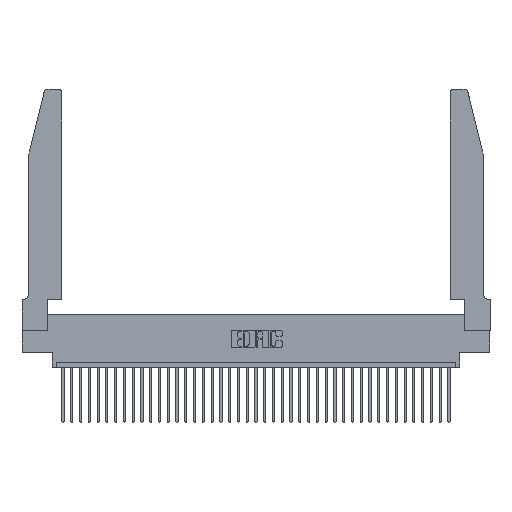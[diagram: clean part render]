
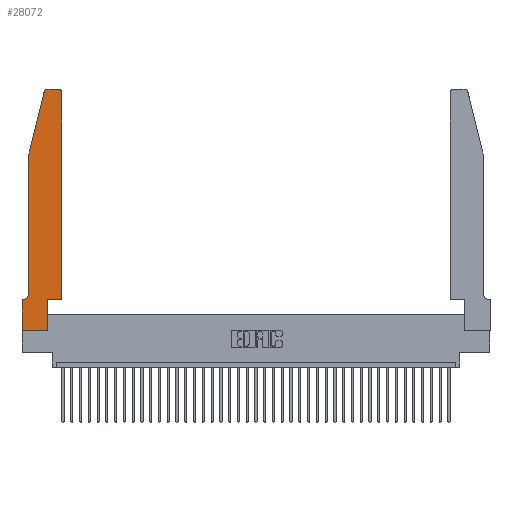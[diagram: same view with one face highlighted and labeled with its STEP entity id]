
A CAD part, top view. The second image highlights one B-rep face of the part: STEP entity #28072.
In plain terms, the highlighted planar face has unit normal (0, 0, 1).
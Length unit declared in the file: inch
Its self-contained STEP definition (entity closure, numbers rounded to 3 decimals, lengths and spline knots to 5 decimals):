
#357 = LINE ( 'NONE', #16555, #23181 ) ;
#1346 = CIRCLE ( 'NONE', #31957, 0.03 ) ;
#1990 = DIRECTION ( 'NONE',  ( 0., 0., 1. ) ) ;
#2924 = LINE ( 'NONE', #20787, #32673 ) ;
#2944 = VECTOR ( 'NONE', #13005, 39.37008 ) ;
#3031 = CARTESIAN_POINT ( 'NONE',  ( 0.2865, 0.35, 0.37 ) ) ;
#4112 = LINE ( 'NONE', #12819, #25993 ) ;
#4734 = VERTEX_POINT ( 'NONE', #30804 ) ;
#5305 = CARTESIAN_POINT ( 'NONE',  ( 0.4205, 2.72, 0.37 ) ) ;
#6623 = EDGE_CURVE ( 'NONE', #35431, #8746, #32338, .T. ) ;
#6817 = VERTEX_POINT ( 'NONE', #30209 ) ;
#7334 = VERTEX_POINT ( 'NONE', #3031 ) ;
#8746 = VERTEX_POINT ( 'NONE', #32816 ) ;
#8953 = FACE_OUTER_BOUND ( 'NONE', #31572, .T. ) ;
#9364 = VERTEX_POINT ( 'NONE', #17082 ) ;
#9685 = VECTOR ( 'NONE', #36013, 39.37008 ) ;
#10014 = PLANE ( 'NONE',  #37730 ) ;
#10068 = EDGE_CURVE ( 'NONE', #6817, #4734, #2924, .T. ) ;
#10417 = DIRECTION ( 'NONE',  ( -1., 0., 0. ) ) ;
#10592 = DIRECTION ( 'NONE',  ( 1., 0., 0. ) ) ;
#10705 = LINE ( 'NONE', #31469, #27034 ) ;
#11403 = CIRCLE ( 'NONE', #19090, 0.07 ) ;
#11939 = EDGE_CURVE ( 'NONE', #7334, #16787, #18132, .T. ) ;
#12170 = DIRECTION ( 'NONE',  ( 0., -1., 0. ) ) ;
#12819 = CARTESIAN_POINT ( 'NONE',  ( 0., 0., 0.37 ) ) ;
#13005 = DIRECTION ( 'NONE',  ( 0., 1., 0. ) ) ;
#13287 = DIRECTION ( 'NONE',  ( -1., 0., 0. ) ) ;
#14295 = VERTEX_POINT ( 'NONE', #26283 ) ;
#14469 = ORIENTED_EDGE ( 'NONE', *, *, #35152, .T. ) ;
#14645 = EDGE_CURVE ( 'NONE', #8746, #24609, #357, .T. ) ;
#14706 = VECTOR ( 'NONE', #13287, 39.37008 ) ;
#14794 = ORIENTED_EDGE ( 'NONE', *, *, #6623, .T. ) ;
#15460 = CARTESIAN_POINT ( 'NONE',  ( 0., 0., 0.37 ) ) ;
#16555 = CARTESIAN_POINT ( 'NONE',  ( 0.2605, 2.75, 0.37 ) ) ;
#16592 = ORIENTED_EDGE ( 'NONE', *, *, #22029, .T. ) ;
#16787 = VERTEX_POINT ( 'NONE', #27229 ) ;
#17003 = LINE ( 'NONE', #29229, #31862 ) ;
#17082 = CARTESIAN_POINT ( 'NONE',  ( 0.2865, 0., 0.37 ) ) ;
#17412 = DIRECTION ( 'NONE',  ( 0., 1., 0. ) ) ;
#18132 = LINE ( 'NONE', #36549, #33831 ) ;
#18248 = DIRECTION ( 'NONE',  ( 0., 0., -1. ) ) ;
#18869 = DIRECTION ( 'NONE',  ( 1., 0., 0. ) ) ;
#18885 = ORIENTED_EDGE ( 'NONE', *, *, #10068, .T. ) ;
#19090 = AXIS2_PLACEMENT_3D ( 'NONE', #21346, #18248, #27197 ) ;
#19266 = ORIENTED_EDGE ( 'NONE', *, *, #11939, .T. ) ;
#19578 = ORIENTED_EDGE ( 'NONE', *, *, #30444, .T. ) ;
#19778 = CARTESIAN_POINT ( 'NONE',  ( 0.284, 2.72, 0.37 ) ) ;
#20016 = DIRECTION ( 'NONE',  ( 1., 0., 0. ) ) ;
#20787 = CARTESIAN_POINT ( 'NONE',  ( 0.0755, 2., 0.37 ) ) ;
#21346 = CARTESIAN_POINT ( 'NONE',  ( 0.0055, 0.42, 0.37 ) ) ;
#21684 = DIRECTION ( 'NONE',  ( 0., -1., 0. ) ) ;
#22029 = EDGE_CURVE ( 'NONE', #32150, #29102, #4112, .T. ) ;
#22425 = CARTESIAN_POINT ( 'NONE',  ( 0.4505, 2.72, 0.37 ) ) ;
#23181 = VECTOR ( 'NONE', #10417, 39.37008 ) ;
#24096 = AXIS2_PLACEMENT_3D ( 'NONE', #5305, #28846, #20016 ) ;
#24230 = EDGE_CURVE ( 'NONE', #25851, #32150, #30988, .T. ) ;
#24609 = VERTEX_POINT ( 'NONE', #24848 ) ;
#24848 = CARTESIAN_POINT ( 'NONE',  ( 0.284, 2.75, 0.37 ) ) ;
#25157 = ORIENTED_EDGE ( 'NONE', *, *, #29667, .T. ) ;
#25437 = DIRECTION ( 'NONE',  ( 0., 0., 1. ) ) ;
#25612 = DIRECTION ( 'NONE',  ( -0.239, -0.971, 0. ) ) ;
#25772 = DIRECTION ( 'NONE',  ( 1., 0., 0. ) ) ;
#25851 = VERTEX_POINT ( 'NONE', #28996 ) ;
#25986 = LINE ( 'NONE', #15460, #9685 ) ;
#25993 = VECTOR ( 'NONE', #21684, 39.37008 ) ;
#26283 = CARTESIAN_POINT ( 'NONE',  ( 0.25487, 2.72718, 0.37 ) ) ;
#27034 = VECTOR ( 'NONE', #25612, 39.37008 ) ;
#27197 = DIRECTION ( 'NONE',  ( -1., 0., 0. ) ) ;
#27229 = CARTESIAN_POINT ( 'NONE',  ( 0.4505, 0.35, 0.37 ) ) ;
#28047 = ORIENTED_EDGE ( 'NONE', *, *, #24230, .T. ) ;
#28072 = ADVANCED_FACE ( 'NONE', ( #8953 ), #10014, .T. ) ;
#28846 = DIRECTION ( 'NONE',  ( 0., 0., 1. ) ) ;
#28996 = CARTESIAN_POINT ( 'NONE',  ( 0.0055, 0.35, 0.37 ) ) ;
#29102 = VERTEX_POINT ( 'NONE', #34583 ) ;
#29229 = CARTESIAN_POINT ( 'NONE',  ( 0.4505, 0.35, 0.37 ) ) ;
#29553 = CARTESIAN_POINT ( 'NONE',  ( 0., 0.35, 0.37 ) ) ;
#29667 = EDGE_CURVE ( 'NONE', #14295, #6817, #10705, .T. ) ;
#30209 = CARTESIAN_POINT ( 'NONE',  ( 0.0755, 2., 0.37 ) ) ;
#30444 = EDGE_CURVE ( 'NONE', #24609, #14295, #1346, .T. ) ;
#30804 = CARTESIAN_POINT ( 'NONE',  ( 0.0755, 0.42, 0.37 ) ) ;
#30951 = CARTESIAN_POINT ( 'NONE',  ( 0.2865, 0.35, 0.37 ) ) ;
#30988 = LINE ( 'NONE', #36816, #14706 ) ;
#31025 = EDGE_CURVE ( 'NONE', #29102, #9364, #25986, .T. ) ;
#31469 = CARTESIAN_POINT ( 'NONE',  ( 0.0755, 2., 0.37 ) ) ;
#31572 = EDGE_LOOP ( 'NONE', ( #38033, #19578, #25157, #18885, #37430, #28047, #16592, #37583, #34240, #19266, #14469, #14794 ) ) ;
#31862 = VECTOR ( 'NONE', #17412, 39.37008 ) ;
#31957 = AXIS2_PLACEMENT_3D ( 'NONE', #19778, #1990, #25772 ) ;
#32150 = VERTEX_POINT ( 'NONE', #29553 ) ;
#32338 = CIRCLE ( 'NONE', #24096, 0.03 ) ;
#32673 = VECTOR ( 'NONE', #12170, 39.37008 ) ;
#32816 = CARTESIAN_POINT ( 'NONE',  ( 0.4205, 2.75, 0.37 ) ) ;
#33831 = VECTOR ( 'NONE', #18869, 39.37008 ) ;
#34223 = EDGE_CURVE ( 'NONE', #4734, #25851, #11403, .T. ) ;
#34240 = ORIENTED_EDGE ( 'NONE', *, *, #35970, .T. ) ;
#34583 = CARTESIAN_POINT ( 'NONE',  ( 0., 0., 0.37 ) ) ;
#35152 = EDGE_CURVE ( 'NONE', #16787, #35431, #17003, .T. ) ;
#35407 = LINE ( 'NONE', #30951, #2944 ) ;
#35431 = VERTEX_POINT ( 'NONE', #22425 ) ;
#35970 = EDGE_CURVE ( 'NONE', #9364, #7334, #35407, .T. ) ;
#36013 = DIRECTION ( 'NONE',  ( 1., 0., 0. ) ) ;
#36549 = CARTESIAN_POINT ( 'NONE',  ( 0.4505, 0.35, 0.37 ) ) ;
#36816 = CARTESIAN_POINT ( 'NONE',  ( 0.0755, 0.35, 0.37 ) ) ;
#37246 = CARTESIAN_POINT ( 'NONE',  ( 0., 0.35, 0.37 ) ) ;
#37430 = ORIENTED_EDGE ( 'NONE', *, *, #34223, .T. ) ;
#37583 = ORIENTED_EDGE ( 'NONE', *, *, #31025, .T. ) ;
#37730 = AXIS2_PLACEMENT_3D ( 'NONE', #37246, #25437, #10592 ) ;
#38033 = ORIENTED_EDGE ( 'NONE', *, *, #14645, .T. ) ;
